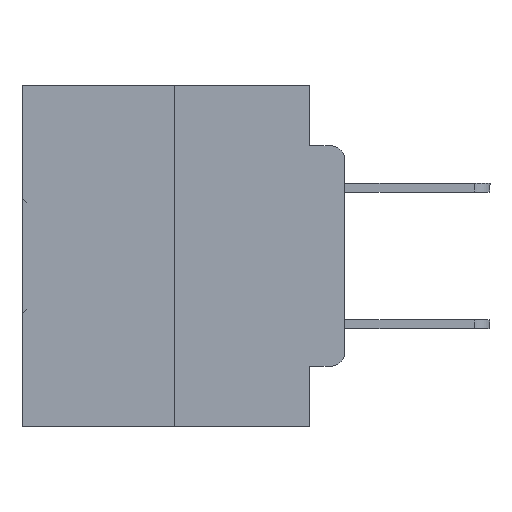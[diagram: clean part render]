
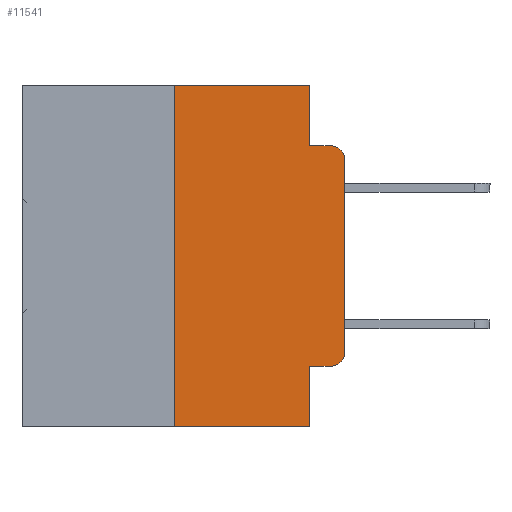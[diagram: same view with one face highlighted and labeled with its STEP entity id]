
A CAD part, left-side view. The second image highlights one B-rep face of the part: STEP entity #11541.
In plain terms, the highlighted planar face has unit normal (-1, 0, 0).
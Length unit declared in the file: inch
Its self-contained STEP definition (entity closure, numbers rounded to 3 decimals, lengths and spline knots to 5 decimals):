
#865 = EDGE_CURVE ( 'NONE', #30531, #5548, #3509, .T. ) ;
#1043 = DIRECTION ( 'NONE',  ( 0., 0., -1. ) ) ;
#2084 = CARTESIAN_POINT ( 'NONE',  ( 0., 0.02, -0.3915 ) ) ;
#2559 = CARTESIAN_POINT ( 'NONE',  ( 0., 0., -0.1085 ) ) ;
#3404 = VECTOR ( 'NONE', #11295, 39.37008 ) ;
#3421 = EDGE_CURVE ( 'NONE', #26539, #14754, #29886, .T. ) ;
#3509 = LINE ( 'NONE', #11932, #22758 ) ;
#4234 = CARTESIAN_POINT ( 'NONE',  ( 0., 0.473, 0. ) ) ;
#4346 = CARTESIAN_POINT ( 'NONE',  ( 0., 0.051, 0. ) ) ;
#4591 = EDGE_CURVE ( 'NONE', #21848, #19415, #20143, .T. ) ;
#4628 = DIRECTION ( 'NONE',  ( 0., 0., -1. ) ) ;
#4757 = AXIS2_PLACEMENT_3D ( 'NONE', #14227, #31409, #16710 ) ;
#4885 = CARTESIAN_POINT ( 'NONE',  ( 0., 0.051, 0. ) ) ;
#5022 = LINE ( 'NONE', #5515, #29955 ) ;
#5338 = CARTESIAN_POINT ( 'NONE',  ( 0., 0.25, 0. ) ) ;
#5515 = CARTESIAN_POINT ( 'NONE',  ( 0., 0.051, -0.4115 ) ) ;
#5548 = VERTEX_POINT ( 'NONE', #2559 ) ;
#6004 = VECTOR ( 'NONE', #22888, 39.37008 ) ;
#6081 = LINE ( 'NONE', #17875, #12038 ) ;
#7545 = ORIENTED_EDGE ( 'NONE', *, *, #16068, .F. ) ;
#8847 = CARTESIAN_POINT ( 'NONE',  ( 0., 0.051, -0.0885 ) ) ;
#9101 = EDGE_LOOP ( 'NONE', ( #16425, #20097, #17410, #12325, #27391, #7545, #24104, #26624, #31555, #21612 ) ) ;
#9234 = VERTEX_POINT ( 'NONE', #5338 ) ;
#9337 = PLANE ( 'NONE',  #16621 ) ;
#10142 = VECTOR ( 'NONE', #1043, 39.37008 ) ;
#11295 = DIRECTION ( 'NONE',  ( 0., -1., 0. ) ) ;
#11498 = EDGE_CURVE ( 'NONE', #5548, #15329, #14176, .T. ) ;
#11541 = ADVANCED_FACE ( 'NONE', ( #12571 ), #9337, .F. ) ;
#11751 = CARTESIAN_POINT ( 'NONE',  ( 0., 0.051, 0. ) ) ;
#11899 = DIRECTION ( 'NONE',  ( 1., 0., 0. ) ) ;
#11932 = CARTESIAN_POINT ( 'NONE',  ( 0., 0., 0. ) ) ;
#11941 = CARTESIAN_POINT ( 'NONE',  ( 0., 0.02, -0.4115 ) ) ;
#12038 = VECTOR ( 'NONE', #20369, 39.37008 ) ;
#12082 = VECTOR ( 'NONE', #32235, 39.37008 ) ;
#12325 = ORIENTED_EDGE ( 'NONE', *, *, #3421, .F. ) ;
#12571 = FACE_OUTER_BOUND ( 'NONE', #9101, .T. ) ;
#12749 = VERTEX_POINT ( 'NONE', #11941 ) ;
#13368 = LINE ( 'NONE', #28886, #25768 ) ;
#13727 = CARTESIAN_POINT ( 'NONE',  ( 0., 0.051, -0.0885 ) ) ;
#13784 = CIRCLE ( 'NONE', #17842, 0.02 ) ;
#14176 = CIRCLE ( 'NONE', #4757, 0.02 ) ;
#14227 = CARTESIAN_POINT ( 'NONE',  ( 0., 0.02, -0.1085 ) ) ;
#14359 = DIRECTION ( 'NONE',  ( 0., 0., 1. ) ) ;
#14497 = EDGE_CURVE ( 'NONE', #28940, #19415, #26707, .T. ) ;
#14754 = VERTEX_POINT ( 'NONE', #8847 ) ;
#14758 = CARTESIAN_POINT ( 'NONE',  ( 0., 0.051, -0.5 ) ) ;
#15329 = VERTEX_POINT ( 'NONE', #18589 ) ;
#16068 = EDGE_CURVE ( 'NONE', #28940, #9234, #13368, .T. ) ;
#16425 = ORIENTED_EDGE ( 'NONE', *, *, #865, .T. ) ;
#16603 = DIRECTION ( 'NONE',  ( 0., 0., 1. ) ) ;
#16621 = AXIS2_PLACEMENT_3D ( 'NONE', #4234, #11899, #29200 ) ;
#16710 = DIRECTION ( 'NONE',  ( 0., 0., -1. ) ) ;
#17410 = ORIENTED_EDGE ( 'NONE', *, *, #30234, .F. ) ;
#17842 = AXIS2_PLACEMENT_3D ( 'NONE', #2084, #19693, #4628 ) ;
#17875 = CARTESIAN_POINT ( 'NONE',  ( 0., 0.473, 0. ) ) ;
#18589 = CARTESIAN_POINT ( 'NONE',  ( 0., 0.02, -0.0885 ) ) ;
#19415 = VERTEX_POINT ( 'NONE', #14758 ) ;
#19693 = DIRECTION ( 'NONE',  ( -1., 0., 0. ) ) ;
#20097 = ORIENTED_EDGE ( 'NONE', *, *, #11498, .T. ) ;
#20143 = LINE ( 'NONE', #4885, #12082 ) ;
#20369 = DIRECTION ( 'NONE',  ( 0., -1., 0. ) ) ;
#20984 = CARTESIAN_POINT ( 'NONE',  ( 0., 0.051, -0.4115 ) ) ;
#21515 = EDGE_CURVE ( 'NONE', #12749, #30531, #13784, .T. ) ;
#21612 = ORIENTED_EDGE ( 'NONE', *, *, #21515, .T. ) ;
#21757 = EDGE_CURVE ( 'NONE', #21848, #12749, #5022, .T. ) ;
#21848 = VERTEX_POINT ( 'NONE', #20984 ) ;
#22758 = VECTOR ( 'NONE', #14359, 39.37008 ) ;
#22888 = DIRECTION ( 'NONE',  ( 0., -1., 0. ) ) ;
#24104 = ORIENTED_EDGE ( 'NONE', *, *, #14497, .T. ) ;
#25536 = DIRECTION ( 'NONE',  ( 0., -1., 0. ) ) ;
#25768 = VECTOR ( 'NONE', #16603, 39.37008 ) ;
#26539 = VERTEX_POINT ( 'NONE', #11751 ) ;
#26624 = ORIENTED_EDGE ( 'NONE', *, *, #4591, .F. ) ;
#26707 = LINE ( 'NONE', #27808, #6004 ) ;
#27391 = ORIENTED_EDGE ( 'NONE', *, *, #28110, .F. ) ;
#27808 = CARTESIAN_POINT ( 'NONE',  ( 0., 0.473, -0.5 ) ) ;
#28064 = CARTESIAN_POINT ( 'NONE',  ( 0., 0.25, -0.5 ) ) ;
#28110 = EDGE_CURVE ( 'NONE', #9234, #26539, #6081, .T. ) ;
#28886 = CARTESIAN_POINT ( 'NONE',  ( 0., 0.25, 0. ) ) ;
#28940 = VERTEX_POINT ( 'NONE', #28064 ) ;
#29200 = DIRECTION ( 'NONE',  ( 0., 0., -1. ) ) ;
#29761 = CARTESIAN_POINT ( 'NONE',  ( 0., 0., -0.3915 ) ) ;
#29886 = LINE ( 'NONE', #4346, #10142 ) ;
#29909 = LINE ( 'NONE', #13727, #3404 ) ;
#29955 = VECTOR ( 'NONE', #25536, 39.37008 ) ;
#30234 = EDGE_CURVE ( 'NONE', #14754, #15329, #29909, .T. ) ;
#30531 = VERTEX_POINT ( 'NONE', #29761 ) ;
#31409 = DIRECTION ( 'NONE',  ( -1., 0., 0. ) ) ;
#31555 = ORIENTED_EDGE ( 'NONE', *, *, #21757, .T. ) ;
#32235 = DIRECTION ( 'NONE',  ( 0., 0., -1. ) ) ;
